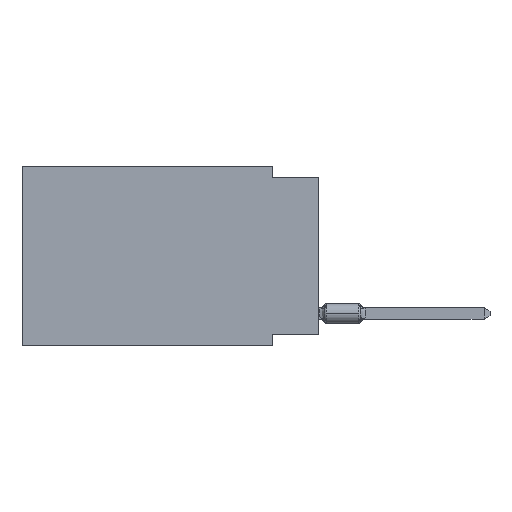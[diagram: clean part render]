
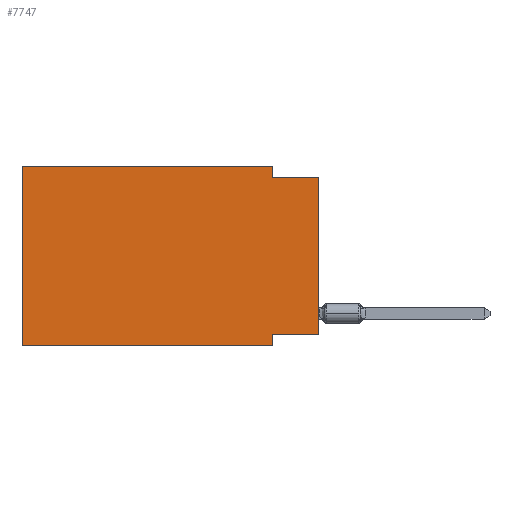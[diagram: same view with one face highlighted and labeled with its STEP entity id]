
A CAD part, left-side view. The second image highlights one B-rep face of the part: STEP entity #7747.
In plain terms, the highlighted planar face has unit normal (-1, 0, 0).
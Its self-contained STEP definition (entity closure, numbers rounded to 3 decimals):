
#83 = VECTOR ( 'NONE', #11928, 1000. ) ;
#279 = VERTEX_POINT ( 'NONE', #1859 ) ;
#341 = CARTESIAN_POINT ( 'NONE',  ( 0., 2.54, -9.906 ) ) ;
#841 = CARTESIAN_POINT ( 'NONE',  ( 0., 16.383, 0. ) ) ;
#1562 = EDGE_CURVE ( 'NONE', #9180, #9564, #7574, .T. ) ;
#1704 = VECTOR ( 'NONE', #2484, 1000. ) ;
#1786 = LINE ( 'NONE', #12935, #6236 ) ;
#1859 = CARTESIAN_POINT ( 'NONE',  ( 0., 2.54, -9.271 ) ) ;
#2252 = EDGE_CURVE ( 'NONE', #9389, #10540, #10495, .T. ) ;
#2276 = CARTESIAN_POINT ( 'NONE',  ( 0., 0., -9.271 ) ) ;
#2484 = DIRECTION ( 'NONE',  ( 0., 0., -1. ) ) ;
#2590 = AXIS2_PLACEMENT_3D ( 'NONE', #14115, #7501, #4369 ) ;
#2728 = DIRECTION ( 'NONE',  ( 0., -1., 0. ) ) ;
#2797 = VECTOR ( 'NONE', #12497, 1000. ) ;
#2878 = EDGE_CURVE ( 'NONE', #9564, #3441, #11112, .T. ) ;
#3022 = EDGE_CURVE ( 'NONE', #3441, #8341, #8379, .T. ) ;
#3369 = FACE_OUTER_BOUND ( 'NONE', #3650, .T. ) ;
#3400 = ORIENTED_EDGE ( 'NONE', *, *, #13731, .F. ) ;
#3441 = VERTEX_POINT ( 'NONE', #13737 ) ;
#3482 = CARTESIAN_POINT ( 'NONE',  ( 0., 0., -0.635 ) ) ;
#3650 = EDGE_LOOP ( 'NONE', ( #14072, #4569, #13941, #6624, #13632, #5462, #4216, #3400 ) ) ;
#3723 = CARTESIAN_POINT ( 'NONE',  ( 0., 16.383, -9.906 ) ) ;
#3773 = CARTESIAN_POINT ( 'NONE',  ( 0., 16.383, -9.906 ) ) ;
#4215 = CARTESIAN_POINT ( 'NONE',  ( 0., 16.383, 0. ) ) ;
#4216 = ORIENTED_EDGE ( 'NONE', *, *, #12740, .F. ) ;
#4369 = DIRECTION ( 'NONE',  ( 0., 0., -1. ) ) ;
#4386 = CARTESIAN_POINT ( 'NONE',  ( 0., 2.54, -9.906 ) ) ;
#4569 = ORIENTED_EDGE ( 'NONE', *, *, #3022, .F. ) ;
#5238 = CARTESIAN_POINT ( 'NONE',  ( 0., 0., -0.635 ) ) ;
#5462 = ORIENTED_EDGE ( 'NONE', *, *, #2252, .T. ) ;
#5839 = VERTEX_POINT ( 'NONE', #11311 ) ;
#5845 = LINE ( 'NONE', #341, #13828 ) ;
#6236 = VECTOR ( 'NONE', #9510, 1000. ) ;
#6624 = ORIENTED_EDGE ( 'NONE', *, *, #1562, .F. ) ;
#6920 = EDGE_CURVE ( 'NONE', #9389, #9180, #10631, .T. ) ;
#7501 = DIRECTION ( 'NONE',  ( 1., 0., 0. ) ) ;
#7574 = LINE ( 'NONE', #11648, #83 ) ;
#7719 = PLANE ( 'NONE',  #2590 ) ;
#7747 = ADVANCED_FACE ( 'NONE', ( #3369 ), #7719, .F. ) ;
#7924 = LINE ( 'NONE', #2276, #12811 ) ;
#8341 = VERTEX_POINT ( 'NONE', #3482 ) ;
#8379 = LINE ( 'NONE', #5238, #11972 ) ;
#8760 = VECTOR ( 'NONE', #2728, 1000. ) ;
#9180 = VERTEX_POINT ( 'NONE', #4215 ) ;
#9389 = VERTEX_POINT ( 'NONE', #3773 ) ;
#9510 = DIRECTION ( 'NONE',  ( 0., 0., 1. ) ) ;
#9564 = VERTEX_POINT ( 'NONE', #10534 ) ;
#9846 = DIRECTION ( 'NONE',  ( 0., 1., 0. ) ) ;
#10045 = CARTESIAN_POINT ( 'NONE',  ( 0., 2.54, 0. ) ) ;
#10495 = LINE ( 'NONE', #3723, #8760 ) ;
#10534 = CARTESIAN_POINT ( 'NONE',  ( 0., 2.54, 0. ) ) ;
#10540 = VERTEX_POINT ( 'NONE', #4386 ) ;
#10631 = LINE ( 'NONE', #841, #2797 ) ;
#11112 = LINE ( 'NONE', #10045, #1704 ) ;
#11145 = EDGE_CURVE ( 'NONE', #5839, #8341, #1786, .T. ) ;
#11311 = CARTESIAN_POINT ( 'NONE',  ( 0., 0., -9.271 ) ) ;
#11400 = DIRECTION ( 'NONE',  ( 0., 0., -1. ) ) ;
#11429 = DIRECTION ( 'NONE',  ( 0., -1., 0. ) ) ;
#11648 = CARTESIAN_POINT ( 'NONE',  ( 0., 16.383, 0. ) ) ;
#11928 = DIRECTION ( 'NONE',  ( 0., -1., 0. ) ) ;
#11972 = VECTOR ( 'NONE', #11429, 1000. ) ;
#12497 = DIRECTION ( 'NONE',  ( 0., 0., 1. ) ) ;
#12740 = EDGE_CURVE ( 'NONE', #279, #10540, #5845, .T. ) ;
#12811 = VECTOR ( 'NONE', #9846, 1000. ) ;
#12935 = CARTESIAN_POINT ( 'NONE',  ( 0., 0., 0. ) ) ;
#13632 = ORIENTED_EDGE ( 'NONE', *, *, #6920, .F. ) ;
#13731 = EDGE_CURVE ( 'NONE', #5839, #279, #7924, .T. ) ;
#13737 = CARTESIAN_POINT ( 'NONE',  ( 0., 2.54, -0.635 ) ) ;
#13828 = VECTOR ( 'NONE', #11400, 1000. ) ;
#13941 = ORIENTED_EDGE ( 'NONE', *, *, #2878, .F. ) ;
#14072 = ORIENTED_EDGE ( 'NONE', *, *, #11145, .T. ) ;
#14115 = CARTESIAN_POINT ( 'NONE',  ( 0., 16.383, 0. ) ) ;
